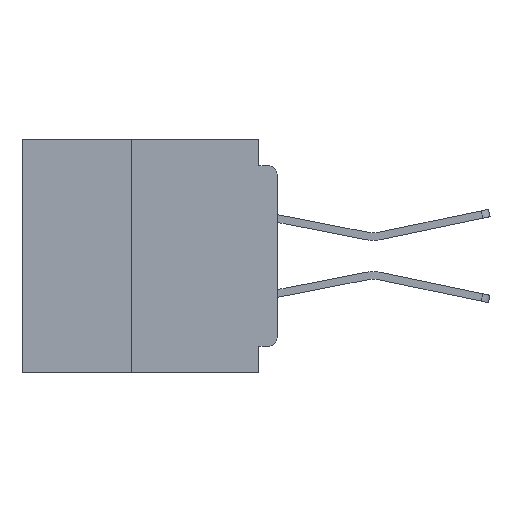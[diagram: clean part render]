
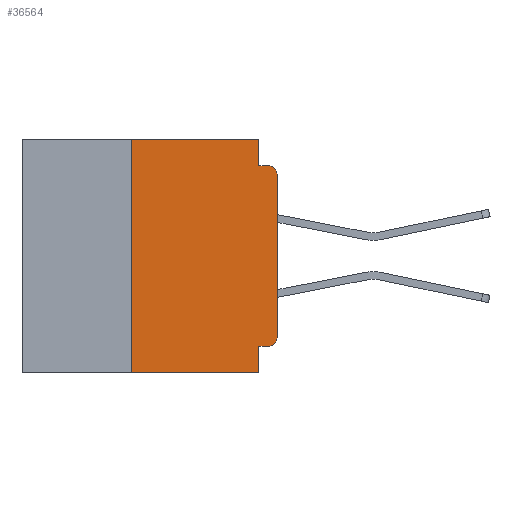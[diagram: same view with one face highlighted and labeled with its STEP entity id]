
A CAD part, left-side view. The second image highlights one B-rep face of the part: STEP entity #36564.
In plain terms, the highlighted planar face has unit normal (-1, 0, 0).
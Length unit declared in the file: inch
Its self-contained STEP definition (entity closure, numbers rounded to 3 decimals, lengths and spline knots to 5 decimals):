
#2032 = VERTEX_POINT ( 'NONE', #48516 ) ;
#2369 = VERTEX_POINT ( 'NONE', #7281 ) ;
#2634 = ORIENTED_EDGE ( 'NONE', *, *, #38481, .F. ) ;
#2698 = ORIENTED_EDGE ( 'NONE', *, *, #14246, .T. ) ;
#3706 = DIRECTION ( 'NONE',  ( 0., 0., -1. ) ) ;
#4550 = CARTESIAN_POINT ( 'NONE',  ( 0., 0.015, -0.34 ) ) ;
#4800 = ORIENTED_EDGE ( 'NONE', *, *, #7030, .T. ) ;
#5490 = CARTESIAN_POINT ( 'NONE',  ( 0., 0.25, -0.4 ) ) ;
#6726 = DIRECTION ( 'NONE',  ( 0., 0., 1. ) ) ;
#6737 = VERTEX_POINT ( 'NONE', #23283 ) ;
#7030 = EDGE_CURVE ( 'NONE', #38659, #25569, #30503, .T. ) ;
#7281 = CARTESIAN_POINT ( 'NONE',  ( 0., 0.031, -0.4 ) ) ;
#7288 = VECTOR ( 'NONE', #3706, 39.37008 ) ;
#8301 = ORIENTED_EDGE ( 'NONE', *, *, #15728, .F. ) ;
#8521 = CARTESIAN_POINT ( 'NONE',  ( 0., 0.437, -0.4 ) ) ;
#8685 = DIRECTION ( 'NONE',  ( 0., 0., -1. ) ) ;
#9423 = CIRCLE ( 'NONE', #10396, 0.015 ) ;
#9938 = CARTESIAN_POINT ( 'NONE',  ( 0., 0., -0.355 ) ) ;
#10396 = AXIS2_PLACEMENT_3D ( 'NONE', #4550, #32928, #8685 ) ;
#10407 = VECTOR ( 'NONE', #48623, 39.37008 ) ;
#10537 = CARTESIAN_POINT ( 'NONE',  ( 0., 0.031, 0. ) ) ;
#11103 = DIRECTION ( 'NONE',  ( 0., 0., -1. ) ) ;
#11251 = ORIENTED_EDGE ( 'NONE', *, *, #23231, .T. ) ;
#11968 = VECTOR ( 'NONE', #14030, 39.37008 ) ;
#12161 = VECTOR ( 'NONE', #6726, 39.37008 ) ;
#13591 = AXIS2_PLACEMENT_3D ( 'NONE', #45741, #21625, #49791 ) ;
#14030 = DIRECTION ( 'NONE',  ( 0., 1., 0. ) ) ;
#14246 = EDGE_CURVE ( 'NONE', #16279, #2369, #31937, .T. ) ;
#14819 = EDGE_LOOP ( 'NONE', ( #4800, #35156, #8301, #19493, #2634, #31501, #2698, #21184, #19036, #11251 ) ) ;
#15728 = EDGE_CURVE ( 'NONE', #2032, #26424, #35646, .T. ) ;
#16279 = VERTEX_POINT ( 'NONE', #5490 ) ;
#16720 = VERTEX_POINT ( 'NONE', #20750 ) ;
#16829 = EDGE_CURVE ( 'NONE', #25569, #26424, #45593, .T. ) ;
#18942 = CARTESIAN_POINT ( 'NONE',  ( 0., 0.015, -0.045 ) ) ;
#19036 = ORIENTED_EDGE ( 'NONE', *, *, #48723, .F. ) ;
#19493 = ORIENTED_EDGE ( 'NONE', *, *, #24163, .F. ) ;
#19784 = VECTOR ( 'NONE', #33121, 39.37008 ) ;
#20750 = CARTESIAN_POINT ( 'NONE',  ( 0., 0.015, -0.355 ) ) ;
#21184 = ORIENTED_EDGE ( 'NONE', *, *, #51871, .F. ) ;
#21625 = DIRECTION ( 'NONE',  ( -1., 0., 0. ) ) ;
#22740 = FACE_OUTER_BOUND ( 'NONE', #14819, .T. ) ;
#22899 = CARTESIAN_POINT ( 'NONE',  ( 0., 0.25, -0.4 ) ) ;
#22958 = CARTESIAN_POINT ( 'NONE',  ( 0., 0.437, 0. ) ) ;
#22959 = LINE ( 'NONE', #22899, #12161 ) ;
#23231 = EDGE_CURVE ( 'NONE', #16720, #38659, #9423, .T. ) ;
#23283 = CARTESIAN_POINT ( 'NONE',  ( 0., 0.25, 0. ) ) ;
#23655 = CARTESIAN_POINT ( 'NONE',  ( 0., 0.031, -0.355 ) ) ;
#24013 = CARTESIAN_POINT ( 'NONE',  ( 0., 0., -0.34 ) ) ;
#24163 = EDGE_CURVE ( 'NONE', #41106, #2032, #48496, .T. ) ;
#24274 = VERTEX_POINT ( 'NONE', #23655 ) ;
#24910 = VECTOR ( 'NONE', #50072, 39.37008 ) ;
#25569 = VERTEX_POINT ( 'NONE', #33114 ) ;
#26424 = VERTEX_POINT ( 'NONE', #18942 ) ;
#27063 = VECTOR ( 'NONE', #34778, 39.37008 ) ;
#30503 = LINE ( 'NONE', #37193, #19784 ) ;
#30625 = VECTOR ( 'NONE', #39176, 39.37008 ) ;
#31308 = PLANE ( 'NONE',  #50694 ) ;
#31501 = ORIENTED_EDGE ( 'NONE', *, *, #39134, .F. ) ;
#31937 = LINE ( 'NONE', #8521, #10407 ) ;
#32928 = DIRECTION ( 'NONE',  ( -1., 0., 0. ) ) ;
#33114 = CARTESIAN_POINT ( 'NONE',  ( 0., 0., -0.06 ) ) ;
#33121 = DIRECTION ( 'NONE',  ( 0., 0., 1. ) ) ;
#33500 = LINE ( 'NONE', #9938, #11968 ) ;
#34778 = DIRECTION ( 'NONE',  ( 0., 0., -1. ) ) ;
#35156 = ORIENTED_EDGE ( 'NONE', *, *, #16829, .T. ) ;
#35353 = DIRECTION ( 'NONE',  ( 1., 0., 0. ) ) ;
#35646 = LINE ( 'NONE', #37960, #24910 ) ;
#36180 = CARTESIAN_POINT ( 'NONE',  ( 0., 0.031, -0.4 ) ) ;
#36564 = ADVANCED_FACE ( 'NONE', ( #22740 ), #31308, .F. ) ;
#37193 = CARTESIAN_POINT ( 'NONE',  ( 0., 0., 0. ) ) ;
#37960 = CARTESIAN_POINT ( 'NONE',  ( 0., 0., -0.045 ) ) ;
#38481 = EDGE_CURVE ( 'NONE', #6737, #41106, #41343, .T. ) ;
#38659 = VERTEX_POINT ( 'NONE', #24013 ) ;
#39134 = EDGE_CURVE ( 'NONE', #16279, #6737, #22959, .T. ) ;
#39176 = DIRECTION ( 'NONE',  ( 0., -1., 0. ) ) ;
#39420 = CARTESIAN_POINT ( 'NONE',  ( 0., 0.031, 0. ) ) ;
#41106 = VERTEX_POINT ( 'NONE', #39420 ) ;
#41343 = LINE ( 'NONE', #22958, #30625 ) ;
#45593 = CIRCLE ( 'NONE', #13591, 0.015 ) ;
#45741 = CARTESIAN_POINT ( 'NONE',  ( 0., 0.015, -0.06 ) ) ;
#47294 = CARTESIAN_POINT ( 'NONE',  ( 0., 0.437, 0. ) ) ;
#48496 = LINE ( 'NONE', #10537, #27063 ) ;
#48516 = CARTESIAN_POINT ( 'NONE',  ( 0., 0.031, -0.045 ) ) ;
#48623 = DIRECTION ( 'NONE',  ( 0., -1., 0. ) ) ;
#48723 = EDGE_CURVE ( 'NONE', #16720, #24274, #33500, .T. ) ;
#49013 = LINE ( 'NONE', #36180, #7288 ) ;
#49791 = DIRECTION ( 'NONE',  ( 0., 0., -1. ) ) ;
#50072 = DIRECTION ( 'NONE',  ( 0., -1., 0. ) ) ;
#50694 = AXIS2_PLACEMENT_3D ( 'NONE', #47294, #35353, #11103 ) ;
#51871 = EDGE_CURVE ( 'NONE', #24274, #2369, #49013, .T. ) ;
